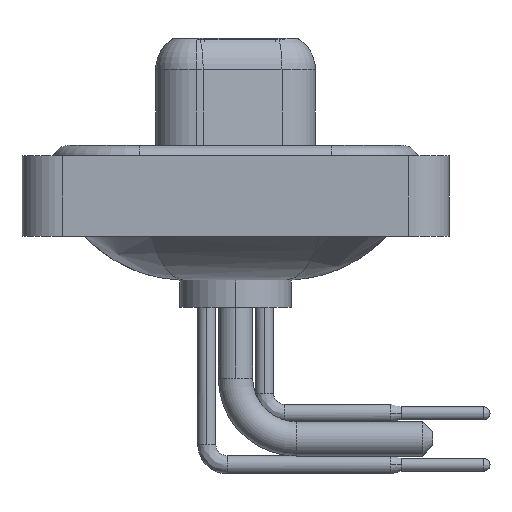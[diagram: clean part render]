
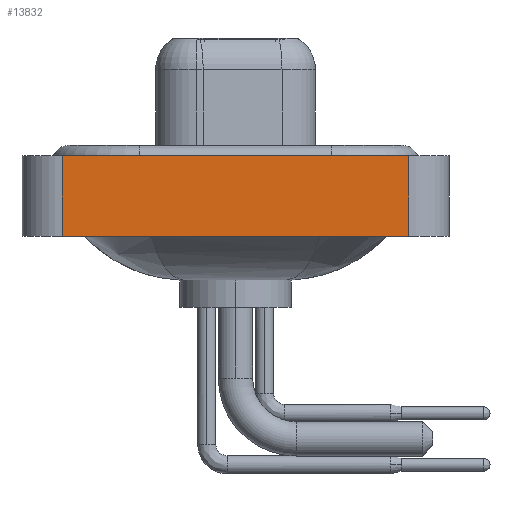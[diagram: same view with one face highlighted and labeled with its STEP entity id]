
A CAD part, left-side view. The second image highlights one B-rep face of the part: STEP entity #13832.
In plain terms, the highlighted planar face has unit normal (-1, 0, 0).
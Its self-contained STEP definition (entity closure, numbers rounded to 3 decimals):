
#441 = VECTOR ( 'NONE', #14036, 1000. ) ;
#846 = LINE ( 'NONE', #9143, #10038 ) ;
#996 = CARTESIAN_POINT ( 'NONE',  ( -7.3, 8.55, -3.6 ) ) ;
#2051 = VERTEX_POINT ( 'NONE', #13731 ) ;
#2490 = LINE ( 'NONE', #7845, #16585 ) ;
#2630 = VERTEX_POINT ( 'NONE', #9824 ) ;
#4308 = VECTOR ( 'NONE', #5456, 1000. ) ;
#5456 = DIRECTION ( 'NONE',  ( 0., 0., 1. ) ) ;
#6564 = EDGE_CURVE ( 'NONE', #17457, #2630, #2490, .T. ) ;
#7269 = DIRECTION ( 'NONE',  ( 0., -1., 0. ) ) ;
#7305 = AXIS2_PLACEMENT_3D ( 'NONE', #19249, #11462, #8335 ) ;
#7845 = CARTESIAN_POINT ( 'NONE',  ( -7.3, -8.55, -3.6 ) ) ;
#8335 = DIRECTION ( 'NONE',  ( 0., 0., 1. ) ) ;
#8993 = LINE ( 'NONE', #996, #4308 ) ;
#9041 = CARTESIAN_POINT ( 'NONE',  ( -7.3, -8.55, -3.6 ) ) ;
#9143 = CARTESIAN_POINT ( 'NONE',  ( -7.3, -8.55, 0.4 ) ) ;
#9824 = CARTESIAN_POINT ( 'NONE',  ( -7.3, -8.55, -3.6 ) ) ;
#10006 = EDGE_CURVE ( 'NONE', #2630, #2051, #12380, .T. ) ;
#10038 = VECTOR ( 'NONE', #7269, 1000. ) ;
#10714 = EDGE_LOOP ( 'NONE', ( #12599, #19879, #18257, #17131 ) ) ;
#11462 = DIRECTION ( 'NONE',  ( -1., 0., 0. ) ) ;
#12340 = CARTESIAN_POINT ( 'NONE',  ( -7.3, 8.55, -3.6 ) ) ;
#12380 = LINE ( 'NONE', #9041, #441 ) ;
#12599 = ORIENTED_EDGE ( 'NONE', *, *, #10006, .T. ) ;
#12922 = FACE_OUTER_BOUND ( 'NONE', #10714, .T. ) ;
#13731 = CARTESIAN_POINT ( 'NONE',  ( -7.3, -8.55, 0.4 ) ) ;
#13832 = ADVANCED_FACE ( 'NONE', ( #12922 ), #16138, .T. ) ;
#14036 = DIRECTION ( 'NONE',  ( 0., 0., 1. ) ) ;
#15293 = CARTESIAN_POINT ( 'NONE',  ( -7.3, 8.55, 0.4 ) ) ;
#15669 = DIRECTION ( 'NONE',  ( 0., -1., 0. ) ) ;
#15867 = EDGE_CURVE ( 'NONE', #17457, #18885, #8993, .T. ) ;
#16138 = PLANE ( 'NONE',  #7305 ) ;
#16585 = VECTOR ( 'NONE', #15669, 1000. ) ;
#17131 = ORIENTED_EDGE ( 'NONE', *, *, #6564, .T. ) ;
#17457 = VERTEX_POINT ( 'NONE', #12340 ) ;
#18257 = ORIENTED_EDGE ( 'NONE', *, *, #15867, .F. ) ;
#18802 = EDGE_CURVE ( 'NONE', #18885, #2051, #846, .T. ) ;
#18885 = VERTEX_POINT ( 'NONE', #15293 ) ;
#19249 = CARTESIAN_POINT ( 'NONE',  ( -7.3, -8.55, -3.6 ) ) ;
#19879 = ORIENTED_EDGE ( 'NONE', *, *, #18802, .F. ) ;
